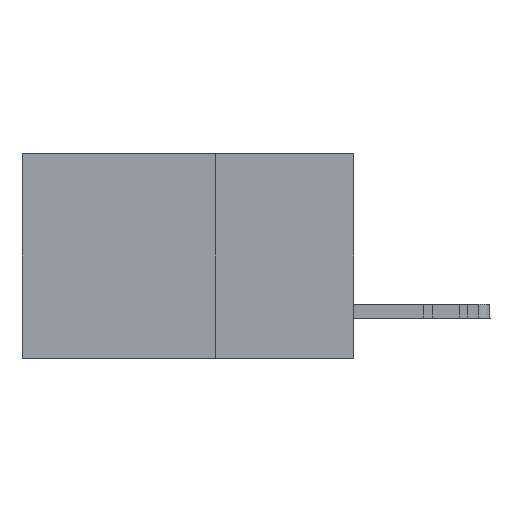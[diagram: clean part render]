
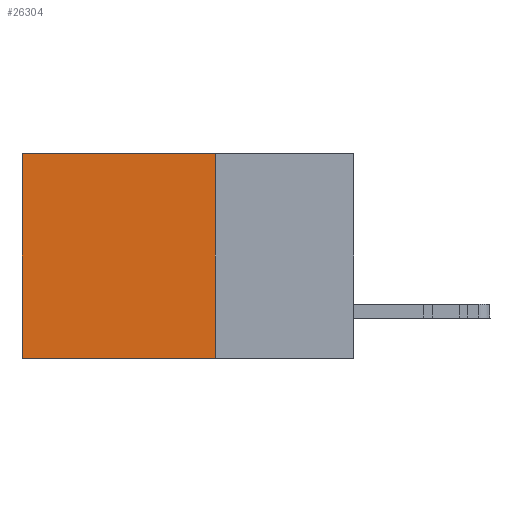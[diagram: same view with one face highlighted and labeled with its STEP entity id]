
A CAD part, left-side view. The second image highlights one B-rep face of the part: STEP entity #26304.
In plain terms, the highlighted planar face has unit normal (-1, 0, 0).
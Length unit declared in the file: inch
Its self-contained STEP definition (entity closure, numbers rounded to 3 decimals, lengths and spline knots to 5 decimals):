
#377 = CARTESIAN_POINT ( 'NONE',  ( 0.2875, 0.6, 0. ) ) ;
#1293 = CARTESIAN_POINT ( 'NONE',  ( 0.2875, 0.25, 0. ) ) ;
#2948 = CARTESIAN_POINT ( 'NONE',  ( 0.2875, 0.25, -0.37 ) ) ;
#5136 = ORIENTED_EDGE ( 'NONE', *, *, #6251, .F. ) ;
#5908 = VERTEX_POINT ( 'NONE', #22550 ) ;
#6251 = EDGE_CURVE ( 'NONE', #24407, #5908, #24242, .T. ) ;
#6375 = EDGE_CURVE ( 'NONE', #5908, #10020, #16116, .T. ) ;
#9576 = PLANE ( 'NONE',  #35103 ) ;
#10020 = VERTEX_POINT ( 'NONE', #38017 ) ;
#10160 = LINE ( 'NONE', #377, #14136 ) ;
#10918 = LINE ( 'NONE', #29863, #22732 ) ;
#14136 = VECTOR ( 'NONE', #16736, 39.37008 ) ;
#16116 = LINE ( 'NONE', #2948, #31514 ) ;
#16308 = ORIENTED_EDGE ( 'NONE', *, *, #6375, .F. ) ;
#16358 = DIRECTION ( 'NONE',  ( 0., 0., -1. ) ) ;
#16736 = DIRECTION ( 'NONE',  ( 0., 0., -1. ) ) ;
#22550 = CARTESIAN_POINT ( 'NONE',  ( 0.2875, 0.25, -0.37 ) ) ;
#22732 = VECTOR ( 'NONE', #30501, 39.37008 ) ;
#24242 = LINE ( 'NONE', #1293, #25407 ) ;
#24394 = EDGE_CURVE ( 'NONE', #24407, #36062, #10918, .T. ) ;
#24407 = VERTEX_POINT ( 'NONE', #33054 ) ;
#25407 = VECTOR ( 'NONE', #40840, 39.37008 ) ;
#25747 = CARTESIAN_POINT ( 'NONE',  ( 0.2875, 0.25, 0. ) ) ;
#26304 = ADVANCED_FACE ( 'NONE', ( #38722 ), #9576, .F. ) ;
#27176 = CARTESIAN_POINT ( 'NONE',  ( 0.2875, 0.6, 0. ) ) ;
#28226 = EDGE_CURVE ( 'NONE', #36062, #10020, #10160, .T. ) ;
#28487 = DIRECTION ( 'NONE',  ( 0., 1., 0. ) ) ;
#28523 = DIRECTION ( 'NONE',  ( 1., 0., 0. ) ) ;
#29863 = CARTESIAN_POINT ( 'NONE',  ( 0.2875, 0.25, 0. ) ) ;
#30501 = DIRECTION ( 'NONE',  ( 0., 1., 0. ) ) ;
#30850 = ORIENTED_EDGE ( 'NONE', *, *, #24394, .T. ) ;
#31249 = ORIENTED_EDGE ( 'NONE', *, *, #28226, .T. ) ;
#31514 = VECTOR ( 'NONE', #28487, 39.37008 ) ;
#33054 = CARTESIAN_POINT ( 'NONE',  ( 0.2875, 0.25, 0. ) ) ;
#35103 = AXIS2_PLACEMENT_3D ( 'NONE', #25747, #28523, #16358 ) ;
#36062 = VERTEX_POINT ( 'NONE', #27176 ) ;
#38017 = CARTESIAN_POINT ( 'NONE',  ( 0.2875, 0.6, -0.37 ) ) ;
#38463 = EDGE_LOOP ( 'NONE', ( #31249, #16308, #5136, #30850 ) ) ;
#38722 = FACE_OUTER_BOUND ( 'NONE', #38463, .T. ) ;
#40840 = DIRECTION ( 'NONE',  ( 0., 0., -1. ) ) ;
